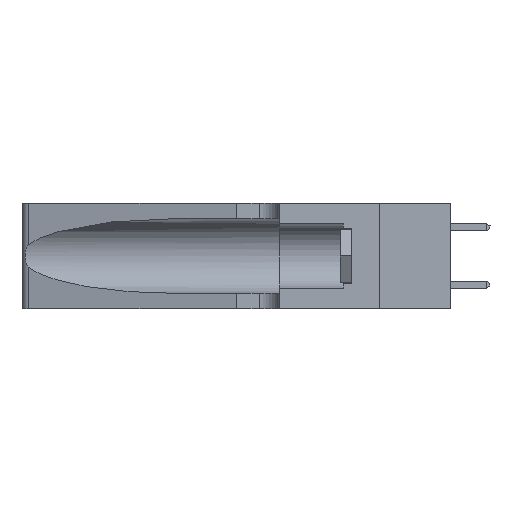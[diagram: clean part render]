
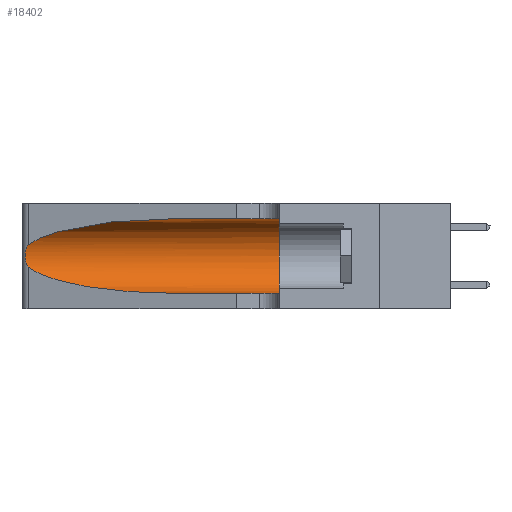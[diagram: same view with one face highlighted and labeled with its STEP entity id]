
A CAD part, left-side view. The second image highlights one B-rep face of the part: STEP entity #18402.
In plain terms, the highlighted cylindrical face has radius 3.308 mm (diameter 6.617 mm), a partial arc.
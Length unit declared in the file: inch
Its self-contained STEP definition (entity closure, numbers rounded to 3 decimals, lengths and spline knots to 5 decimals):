
#671 = EDGE_CURVE ( 'NONE', #6515, #15368, #44121, .T. ) ;
#849 = VERTEX_POINT ( 'NONE', #2765 ) ;
#1514 = CARTESIAN_POINT ( 'NONE',  ( 0.26075, 1.23896, 0.178 ) ) ;
#1842 = CARTESIAN_POINT ( 'NONE',  ( 0.18966, 0.96281, 0.31525 ) ) ;
#2765 = CARTESIAN_POINT ( 'NONE',  ( 0.1305, 0.35, 0.31525 ) ) ;
#2901 = LINE ( 'NONE', #44881, #38730 ) ;
#3707 = DIRECTION ( 'NONE',  ( 0., 1., 0. ) ) ;
#5027 = CARTESIAN_POINT ( 'NONE',  ( 0.25856, 1.23593, 0.16098 ) ) ;
#6515 = VERTEX_POINT ( 'NONE', #6727 ) ;
#6727 = CARTESIAN_POINT ( 'NONE',  ( 0.1305, 0.72297, 0.31525 ) ) ;
#7218 = CARTESIAN_POINT ( 'NONE',  ( 0.25487, 1.22718, 0.14631 ) ) ;
#7421 = AXIS2_PLACEMENT_3D ( 'NONE', #24567, #3707, #28030 ) ;
#8382 = CARTESIAN_POINT ( 'NONE',  ( 0.25555, 1.22994, 0.2215 ) ) ;
#8523 = CARTESIAN_POINT ( 'NONE',  ( 0.25639, 1.23186, 0.15144 ) ) ;
#9171 = ORIENTED_EDGE ( 'NONE', *, *, #671, .T. ) ;
#9859 = CARTESIAN_POINT ( 'NONE',  ( 0.1305, 1.61858, 0.185 ) ) ;
#10713 = CARTESIAN_POINT ( 'NONE',  ( 0.18966, 0.96281, 0.05475 ) ) ;
#10786 = ORIENTED_EDGE ( 'NONE', *, *, #26605, .T. ) ;
#11915 = CARTESIAN_POINT ( 'NONE',  ( 0.25487, 1.22718, 0.22369 ) ) ;
#11929 = B_SPLINE_CURVE_WITH_KNOTS ( 'NONE', 3,
 ( #11915, #8382, #15416, #39624, #18900, #43067, #22411, #1514, #25878, #5027, #29348, #8523, #32833, #12062 ),
 .UNSPECIFIED., .F., .F.,
 ( 4, 2, 2, 2, 2, 2, 4 ),
 ( 0., 0.00027, 0.00053, 0.00107, 0.0016, 0.00187, 0.00214 ),
 .UNSPECIFIED. ) ;
#12062 = CARTESIAN_POINT ( 'NONE',  ( 0.25487, 1.22718, 0.14631 ) ) ;
#14262 = EDGE_CURVE ( 'NONE', #16225, #38881, #41474, .T. ) ;
#15368 = VERTEX_POINT ( 'NONE', #23104 ) ;
#15416 = CARTESIAN_POINT ( 'NONE',  ( 0.25639, 1.23184, 0.21858 ) ) ;
#16225 = VERTEX_POINT ( 'NONE', #24700 ) ;
#16231 = ORIENTED_EDGE ( 'NONE', *, *, #14262, .T. ) ;
#16707 = FACE_OUTER_BOUND ( 'NONE', #29868, .T. ) ;
#17236 = ORIENTED_EDGE ( 'NONE', *, *, #27479, .F. ) ;
#17385 = DIRECTION ( 'NONE',  ( 0., -1., 0. ) ) ;
#18402 = ADVANCED_FACE ( 'NONE', ( #16707 ), #34040, .F. ) ;
#18900 = CARTESIAN_POINT ( 'NONE',  ( 0.25854, 1.2359, 0.20912 ) ) ;
#18918 = ORIENTED_EDGE ( 'NONE', *, *, #26589, .F. ) ;
#19433 = CARTESIAN_POINT ( 'NONE',  ( 0.25487, 1.22718, 0.14631 ) ) ;
#19514 = EDGE_CURVE ( 'NONE', #15368, #22078, #11929, .T. ) ;
#22078 = VERTEX_POINT ( 'NONE', #19433 ) ;
#22411 = CARTESIAN_POINT ( 'NONE',  ( 0.26075, 1.23896, 0.19203 ) ) ;
#22727 = CARTESIAN_POINT ( 'NONE',  ( 0.2373, 1.15595, 0.28018 ) ) ;
#23104 = CARTESIAN_POINT ( 'NONE',  ( 0.25487, 1.22718, 0.22369 ) ) ;
#23721 = DIRECTION ( 'NONE',  ( 0., -1., 0. ) ) ;
#24421 = AXIS2_PLACEMENT_3D ( 'NONE', #9859, #23721, #27186 ) ;
#24567 = CARTESIAN_POINT ( 'NONE',  ( 0.1305, 0.35, 0.185 ) ) ;
#24700 = CARTESIAN_POINT ( 'NONE',  ( 0.1305, 0.72297, 0.05475 ) ) ;
#25878 = CARTESIAN_POINT ( 'NONE',  ( 0.26017, 1.23833, 0.17102 ) ) ;
#26198 = CARTESIAN_POINT ( 'NONE',  ( 0.1305, 0.72297, 0.31525 ) ) ;
#26589 = EDGE_CURVE ( 'NONE', #849, #38881, #39894, .T. ) ;
#26605 = EDGE_CURVE ( 'NONE', #22078, #16225, #32779, .T. ) ;
#27186 = DIRECTION ( 'NONE',  ( 0., 0., -1. ) ) ;
#27479 = EDGE_CURVE ( 'NONE', #6515, #849, #2901, .T. ) ;
#27683 = CARTESIAN_POINT ( 'NONE',  ( 0.1305, 1.61858, 0.05475 ) ) ;
#28030 = DIRECTION ( 'NONE',  ( 0., 0., 1. ) ) ;
#29348 = CARTESIAN_POINT ( 'NONE',  ( 0.25789, 1.23486, 0.15765 ) ) ;
#29664 = CARTESIAN_POINT ( 'NONE',  ( 0.25487, 1.22718, 0.22369 ) ) ;
#29868 = EDGE_LOOP ( 'NONE', ( #9171, #41691, #10786, #16231, #18918, #17236 ) ) ;
#30133 = VECTOR ( 'NONE', #41554, 39.37008 ) ;
#31508 = CARTESIAN_POINT ( 'NONE',  ( 0.2373, 1.15595, 0.08982 ) ) ;
#32779 =( BOUNDED_CURVE ( )  B_SPLINE_CURVE ( 3, ( #7218, #31508, #10713, #34993 ),
 .UNSPECIFIED., .F., .F. ) 
 B_SPLINE_CURVE_WITH_KNOTS ( ( 4, 4 ),
 ( 3.44316, 4.71239 ),
 .UNSPECIFIED. ) 
 CURVE ( )  GEOMETRIC_REPRESENTATION_ITEM ( )  RATIONAL_B_SPLINE_CURVE ( ( 1., 0.87, 0.87, 1. ) ) 
 REPRESENTATION_ITEM ( '' )  );
#32833 = CARTESIAN_POINT ( 'NONE',  ( 0.25555, 1.22993, 0.14849 ) ) ;
#34040 = CYLINDRICAL_SURFACE ( 'NONE', #24421, 0.13025 ) ;
#34993 = CARTESIAN_POINT ( 'NONE',  ( 0.1305, 0.72297, 0.05475 ) ) ;
#35928 = CARTESIAN_POINT ( 'NONE',  ( 0.1305, 0.35, 0.05475 ) ) ;
#38730 = VECTOR ( 'NONE', #17385, 39.37008 ) ;
#38881 = VERTEX_POINT ( 'NONE', #35928 ) ;
#39624 = CARTESIAN_POINT ( 'NONE',  ( 0.25787, 1.23484, 0.2124 ) ) ;
#39894 = CIRCLE ( 'NONE', #7421, 0.13025 ) ;
#41474 = LINE ( 'NONE', #27683, #30133 ) ;
#41554 = DIRECTION ( 'NONE',  ( 0., -1., 0. ) ) ;
#41691 = ORIENTED_EDGE ( 'NONE', *, *, #19514, .T. ) ;
#43067 = CARTESIAN_POINT ( 'NONE',  ( 0.26018, 1.23835, 0.19895 ) ) ;
#44121 =( BOUNDED_CURVE ( )  B_SPLINE_CURVE ( 3, ( #26198, #1842, #22727, #29664 ),
 .UNSPECIFIED., .F., .F. ) 
 B_SPLINE_CURVE_WITH_KNOTS ( ( 4, 4 ),
 ( 1.5708, 2.84003 ),
 .UNSPECIFIED. ) 
 CURVE ( )  GEOMETRIC_REPRESENTATION_ITEM ( )  RATIONAL_B_SPLINE_CURVE ( ( 1., 0.87, 0.87, 1. ) ) 
 REPRESENTATION_ITEM ( '' )  );
#44881 = CARTESIAN_POINT ( 'NONE',  ( 0.1305, 1.61858, 0.31525 ) ) ;
